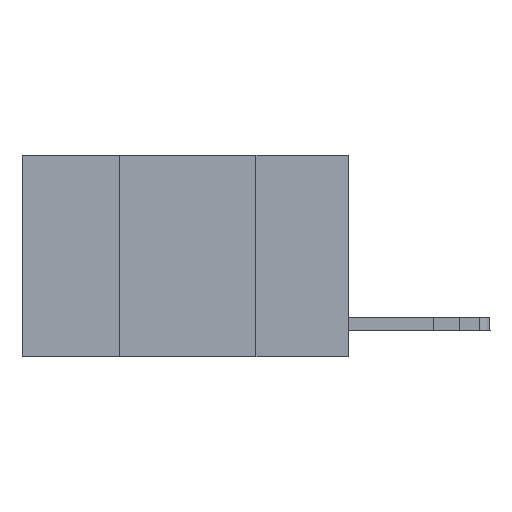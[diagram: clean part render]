
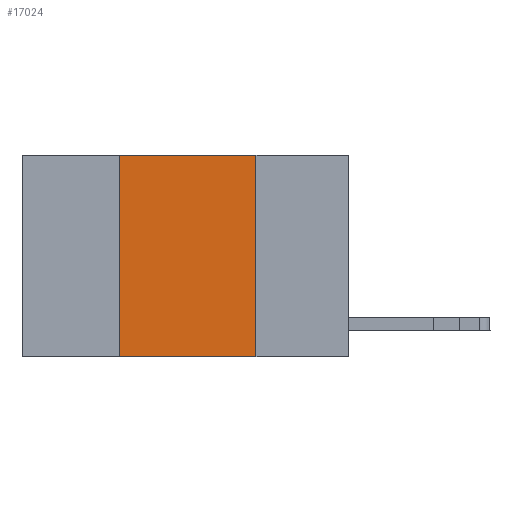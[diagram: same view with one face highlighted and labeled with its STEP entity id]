
A CAD part, left-side view. The second image highlights one B-rep face of the part: STEP entity #17024.
In plain terms, the highlighted planar face has unit normal (-1, 0, 0).
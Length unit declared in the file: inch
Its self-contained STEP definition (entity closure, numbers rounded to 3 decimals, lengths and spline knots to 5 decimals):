
#17 = ORIENTED_EDGE ( 'NONE', *, *, #6323, .F. ) ;
#1224 = EDGE_CURVE ( 'NONE', #2977, #11951, #21711, .T. ) ;
#1277 = PLANE ( 'NONE',  #14627 ) ;
#1352 = LINE ( 'NONE', #5365, #3263 ) ;
#2977 = VERTEX_POINT ( 'NONE', #15624 ) ;
#3263 = VECTOR ( 'NONE', #5228, 39.37008 ) ;
#3546 = DIRECTION ( 'NONE',  ( 0., -1., 0. ) ) ;
#3582 = CARTESIAN_POINT ( 'NONE',  ( 0., 0.6, 0. ) ) ;
#4056 = CARTESIAN_POINT ( 'NONE',  ( 0., 0.17, -0.37 ) ) ;
#4245 = CARTESIAN_POINT ( 'NONE',  ( 0., 0.17, 0. ) ) ;
#5228 = DIRECTION ( 'NONE',  ( 0., 0., 1. ) ) ;
#5365 = CARTESIAN_POINT ( 'NONE',  ( 0., 0.42, 0. ) ) ;
#5528 = DIRECTION ( 'NONE',  ( 0., 0., -1. ) ) ;
#6308 = DIRECTION ( 'NONE',  ( 0., 0., -1. ) ) ;
#6323 = EDGE_CURVE ( 'NONE', #23614, #2977, #21151, .T. ) ;
#7421 = VECTOR ( 'NONE', #6308, 39.37008 ) ;
#8845 = EDGE_LOOP ( 'NONE', ( #16172, #17, #19921, #22823 ) ) ;
#10256 = VECTOR ( 'NONE', #16346, 39.37008 ) ;
#10859 = EDGE_CURVE ( 'NONE', #18354, #23614, #1352, .T. ) ;
#11271 = CARTESIAN_POINT ( 'NONE',  ( 0., 0.6, 0. ) ) ;
#11951 = VERTEX_POINT ( 'NONE', #4056 ) ;
#12498 = CARTESIAN_POINT ( 'NONE',  ( 0., 0.42, 0. ) ) ;
#13002 = CARTESIAN_POINT ( 'NONE',  ( 0., 0.6, -0.37 ) ) ;
#14311 = EDGE_CURVE ( 'NONE', #18354, #11951, #14918, .T. ) ;
#14627 = AXIS2_PLACEMENT_3D ( 'NONE', #3582, #23096, #5528 ) ;
#14918 = LINE ( 'NONE', #13002, #10256 ) ;
#15624 = CARTESIAN_POINT ( 'NONE',  ( 0., 0.17, 0. ) ) ;
#16172 = ORIENTED_EDGE ( 'NONE', *, *, #1224, .F. ) ;
#16346 = DIRECTION ( 'NONE',  ( 0., -1., 0. ) ) ;
#17024 = ADVANCED_FACE ( 'NONE', ( #18914 ), #1277, .F. ) ;
#17366 = CARTESIAN_POINT ( 'NONE',  ( 0., 0.42, -0.37 ) ) ;
#17812 = VECTOR ( 'NONE', #3546, 39.37008 ) ;
#18354 = VERTEX_POINT ( 'NONE', #17366 ) ;
#18914 = FACE_OUTER_BOUND ( 'NONE', #8845, .T. ) ;
#19921 = ORIENTED_EDGE ( 'NONE', *, *, #10859, .F. ) ;
#21151 = LINE ( 'NONE', #11271, #17812 ) ;
#21711 = LINE ( 'NONE', #4245, #7421 ) ;
#22823 = ORIENTED_EDGE ( 'NONE', *, *, #14311, .T. ) ;
#23096 = DIRECTION ( 'NONE',  ( 1., 0., 0. ) ) ;
#23614 = VERTEX_POINT ( 'NONE', #12498 ) ;
